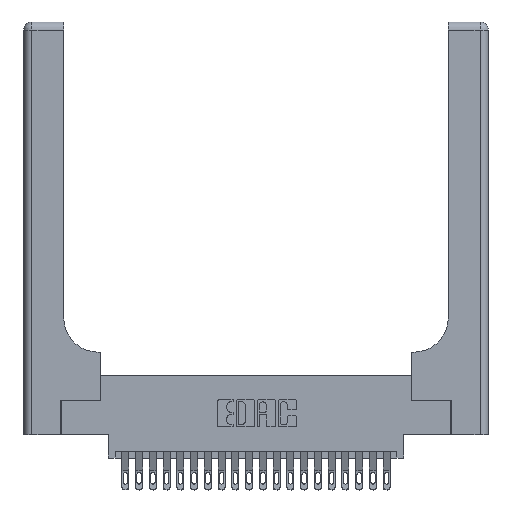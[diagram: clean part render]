
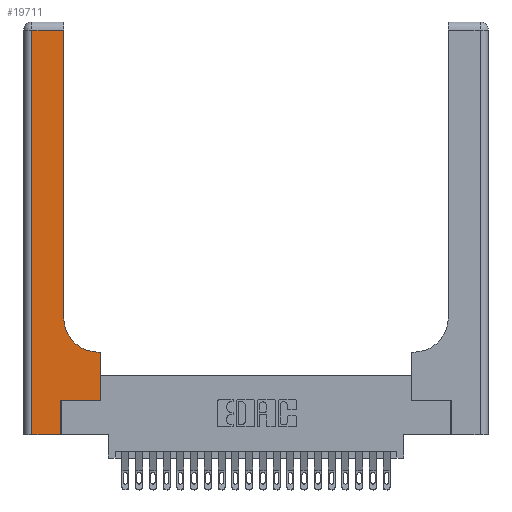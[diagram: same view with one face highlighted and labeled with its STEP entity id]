
A CAD part, top view. The second image highlights one B-rep face of the part: STEP entity #19711.
In plain terms, the highlighted planar face has unit normal (0, 0, 1).
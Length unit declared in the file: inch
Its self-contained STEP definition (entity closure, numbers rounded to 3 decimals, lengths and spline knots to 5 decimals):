
#100 = CARTESIAN_POINT ( 'NONE',  ( 0.5415, 0.6, 0.37 ) ) ;
#508 = VERTEX_POINT ( 'NONE', #100 ) ;
#519 = VERTEX_POINT ( 'NONE', #16013 ) ;
#595 = DIRECTION ( 'NONE',  ( 0., 1., 0. ) ) ;
#622 = DIRECTION ( 'NONE',  ( -1., 0., 0. ) ) ;
#1210 = CARTESIAN_POINT ( 'NONE',  ( 0.06, 2.94, 0.37 ) ) ;
#1386 = CARTESIAN_POINT ( 'NONE',  ( 0.2915, 3., 0.37 ) ) ;
#1495 = ORIENTED_EDGE ( 'NONE', *, *, #1538, .T. ) ;
#1538 = EDGE_CURVE ( 'NONE', #16831, #3606, #6410, .T. ) ;
#1641 = ORIENTED_EDGE ( 'NONE', *, *, #16807, .T. ) ;
#1668 = VECTOR ( 'NONE', #6241, 39.37008 ) ;
#2590 = EDGE_CURVE ( 'NONE', #19152, #15677, #23830, .T. ) ;
#2892 = DIRECTION ( 'NONE',  ( -1., 0., 0. ) ) ;
#3606 = VERTEX_POINT ( 'NONE', #7861 ) ;
#4467 = CARTESIAN_POINT ( 'NONE',  ( 0.269, 0., 0.37 ) ) ;
#4549 = CARTESIAN_POINT ( 'NONE',  ( 0.269, 0.25, 0.37 ) ) ;
#4744 = PLANE ( 'NONE',  #10435 ) ;
#5091 = CARTESIAN_POINT ( 'NONE',  ( 0.5585, 0.25, 0.37 ) ) ;
#5213 = VECTOR ( 'NONE', #17480, 39.37008 ) ;
#5214 = VECTOR ( 'NONE', #18417, 39.37008 ) ;
#6241 = DIRECTION ( 'NONE',  ( 1., 0., 0. ) ) ;
#6244 = CARTESIAN_POINT ( 'NONE',  ( 0.5585, 0.25, 0.37 ) ) ;
#6410 = LINE ( 'NONE', #7203, #12592 ) ;
#6415 = ORIENTED_EDGE ( 'NONE', *, *, #23995, .T. ) ;
#6787 = LINE ( 'NONE', #19362, #1668 ) ;
#7016 = DIRECTION ( 'NONE',  ( 0., 1., 0. ) ) ;
#7203 = CARTESIAN_POINT ( 'NONE',  ( 0., 0., 0.37 ) ) ;
#7320 = DIRECTION ( 'NONE',  ( 0., 0., -1. ) ) ;
#7415 = DIRECTION ( 'NONE',  ( 1., 0., 0. ) ) ;
#7861 = CARTESIAN_POINT ( 'NONE',  ( 0.269, 0., 0.37 ) ) ;
#8197 = EDGE_LOOP ( 'NONE', ( #6415, #20302, #10316, #1495, #9906, #18400, #9386, #1641, #13255 ) ) ;
#8234 = CARTESIAN_POINT ( 'NONE',  ( 0., 2.94, 0.37 ) ) ;
#8427 = VECTOR ( 'NONE', #7016, 39.37008 ) ;
#9056 = LINE ( 'NONE', #4467, #22727 ) ;
#9200 = EDGE_CURVE ( 'NONE', #11685, #17336, #6787, .T. ) ;
#9386 = ORIENTED_EDGE ( 'NONE', *, *, #18573, .T. ) ;
#9906 = ORIENTED_EDGE ( 'NONE', *, *, #13476, .T. ) ;
#10166 = CARTESIAN_POINT ( 'NONE',  ( 0.5585, 0.6, 0.37 ) ) ;
#10316 = ORIENTED_EDGE ( 'NONE', *, *, #12155, .T. ) ;
#10416 = CARTESIAN_POINT ( 'NONE',  ( 0.2915, 0.6, 0.37 ) ) ;
#10435 = AXIS2_PLACEMENT_3D ( 'NONE', #12347, #14250, #2892 ) ;
#11685 = VERTEX_POINT ( 'NONE', #4549 ) ;
#12155 = EDGE_CURVE ( 'NONE', #15677, #16831, #20189, .T. ) ;
#12347 = CARTESIAN_POINT ( 'NONE',  ( 0., 3., 0.37 ) ) ;
#12592 = VECTOR ( 'NONE', #7415, 39.37008 ) ;
#13121 = EDGE_CURVE ( 'NONE', #508, #519, #16713, .T. ) ;
#13255 = ORIENTED_EDGE ( 'NONE', *, *, #13121, .T. ) ;
#13476 = EDGE_CURVE ( 'NONE', #3606, #11685, #9056, .T. ) ;
#14250 = DIRECTION ( 'NONE',  ( 0., 0., -1. ) ) ;
#14597 = CARTESIAN_POINT ( 'NONE',  ( 0.2915, 2.94, 0.37 ) ) ;
#14679 = LINE ( 'NONE', #1386, #5214 ) ;
#15526 = CARTESIAN_POINT ( 'NONE',  ( 0.06, 3., 0.37 ) ) ;
#15677 = VERTEX_POINT ( 'NONE', #1210 ) ;
#16013 = CARTESIAN_POINT ( 'NONE',  ( 0.2915, 0.85, 0.37 ) ) ;
#16024 = AXIS2_PLACEMENT_3D ( 'NONE', #18561, #7320, #20401 ) ;
#16067 = CARTESIAN_POINT ( 'NONE',  ( 0.06, 0., 0.37 ) ) ;
#16713 = CIRCLE ( 'NONE', #16024, 0.25 ) ;
#16807 = EDGE_CURVE ( 'NONE', #21255, #508, #21440, .T. ) ;
#16831 = VERTEX_POINT ( 'NONE', #16067 ) ;
#17135 = VECTOR ( 'NONE', #23373, 39.37008 ) ;
#17336 = VERTEX_POINT ( 'NONE', #6244 ) ;
#17480 = DIRECTION ( 'NONE',  ( 0., -1., 0. ) ) ;
#18400 = ORIENTED_EDGE ( 'NONE', *, *, #9200, .T. ) ;
#18417 = DIRECTION ( 'NONE',  ( 0., 1., 0. ) ) ;
#18561 = CARTESIAN_POINT ( 'NONE',  ( 0.5415, 0.85, 0.37 ) ) ;
#18573 = EDGE_CURVE ( 'NONE', #17336, #21255, #23835, .T. ) ;
#18987 = VECTOR ( 'NONE', #622, 39.37008 ) ;
#19152 = VERTEX_POINT ( 'NONE', #14597 ) ;
#19362 = CARTESIAN_POINT ( 'NONE',  ( 0.269, 0.25, 0.37 ) ) ;
#19711 = ADVANCED_FACE ( 'NONE', ( #20362 ), #4744, .F. ) ;
#20189 = LINE ( 'NONE', #15526, #5213 ) ;
#20302 = ORIENTED_EDGE ( 'NONE', *, *, #2590, .T. ) ;
#20362 = FACE_OUTER_BOUND ( 'NONE', #8197, .T. ) ;
#20401 = DIRECTION ( 'NONE',  ( 1., 0., 0. ) ) ;
#21255 = VERTEX_POINT ( 'NONE', #10166 ) ;
#21440 = LINE ( 'NONE', #10416, #17135 ) ;
#22727 = VECTOR ( 'NONE', #595, 39.37008 ) ;
#23373 = DIRECTION ( 'NONE',  ( -1., 0., 0. ) ) ;
#23830 = LINE ( 'NONE', #8234, #18987 ) ;
#23835 = LINE ( 'NONE', #5091, #8427 ) ;
#23995 = EDGE_CURVE ( 'NONE', #519, #19152, #14679, .T. ) ;
